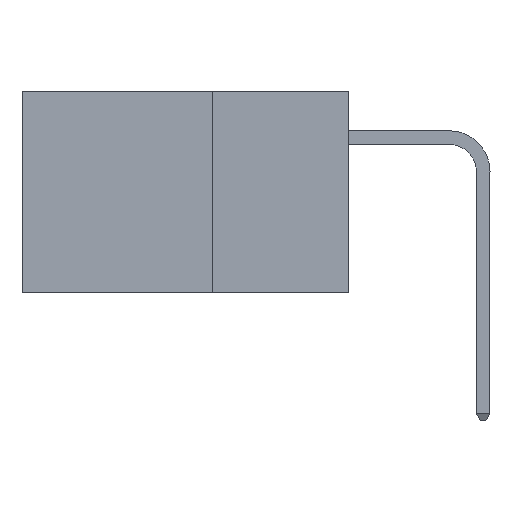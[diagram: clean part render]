
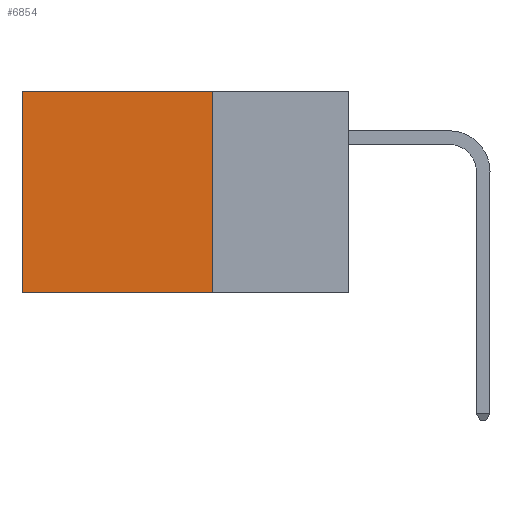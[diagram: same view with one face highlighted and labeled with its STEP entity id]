
A CAD part, left-side view. The second image highlights one B-rep face of the part: STEP entity #6854.
In plain terms, the highlighted planar face has unit normal (-1, 0, 0).
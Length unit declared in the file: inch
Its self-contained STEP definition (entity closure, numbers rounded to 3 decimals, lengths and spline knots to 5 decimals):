
#542 = FACE_OUTER_BOUND ( 'NONE', #11279, .T. ) ;
#1296 = VECTOR ( 'NONE', #21914, 39.37008 ) ;
#1816 = VECTOR ( 'NONE', #30717, 39.37008 ) ;
#2534 = VECTOR ( 'NONE', #22395, 39.37008 ) ;
#3642 = EDGE_CURVE ( 'NONE', #14192, #27919, #27334, .T. ) ;
#4705 = ORIENTED_EDGE ( 'NONE', *, *, #16904, .T. ) ;
#5171 = VERTEX_POINT ( 'NONE', #26095 ) ;
#6854 = ADVANCED_FACE ( 'NONE', ( #542 ), #18082, .F. ) ;
#7007 = VERTEX_POINT ( 'NONE', #25892 ) ;
#8223 = LINE ( 'NONE', #28835, #20538 ) ;
#8258 = DIRECTION ( 'NONE',  ( 0., 0., -1. ) ) ;
#8956 = CARTESIAN_POINT ( 'NONE',  ( 0.2875, 0.25, -0.37 ) ) ;
#11218 = CARTESIAN_POINT ( 'NONE',  ( 0.2875, 0.25, 0. ) ) ;
#11279 = EDGE_LOOP ( 'NONE', ( #28698, #12554, #26484, #4705 ) ) ;
#12554 = ORIENTED_EDGE ( 'NONE', *, *, #3642, .F. ) ;
#14192 = VERTEX_POINT ( 'NONE', #8956 ) ;
#16904 = EDGE_CURVE ( 'NONE', #5171, #7007, #26308, .T. ) ;
#17096 = CARTESIAN_POINT ( 'NONE',  ( 0.2875, 0.6, -0.37 ) ) ;
#18082 = PLANE ( 'NONE',  #29841 ) ;
#18375 = EDGE_CURVE ( 'NONE', #7007, #27919, #8223, .T. ) ;
#20520 = CARTESIAN_POINT ( 'NONE',  ( 0.2875, 0.25, 0. ) ) ;
#20538 = VECTOR ( 'NONE', #31264, 39.37008 ) ;
#21356 = LINE ( 'NONE', #27379, #2534 ) ;
#21914 = DIRECTION ( 'NONE',  ( 0., 1., 0. ) ) ;
#22395 = DIRECTION ( 'NONE',  ( 0., 0., -1. ) ) ;
#22930 = DIRECTION ( 'NONE',  ( 1., 0., 0. ) ) ;
#23438 = EDGE_CURVE ( 'NONE', #5171, #14192, #21356, .T. ) ;
#24254 = CARTESIAN_POINT ( 'NONE',  ( 0.2875, 0.25, -0.37 ) ) ;
#25892 = CARTESIAN_POINT ( 'NONE',  ( 0.2875, 0.6, 0. ) ) ;
#26095 = CARTESIAN_POINT ( 'NONE',  ( 0.2875, 0.25, 0. ) ) ;
#26308 = LINE ( 'NONE', #11218, #1816 ) ;
#26484 = ORIENTED_EDGE ( 'NONE', *, *, #23438, .F. ) ;
#27334 = LINE ( 'NONE', #24254, #1296 ) ;
#27379 = CARTESIAN_POINT ( 'NONE',  ( 0.2875, 0.25, 0. ) ) ;
#27919 = VERTEX_POINT ( 'NONE', #17096 ) ;
#28698 = ORIENTED_EDGE ( 'NONE', *, *, #18375, .T. ) ;
#28835 = CARTESIAN_POINT ( 'NONE',  ( 0.2875, 0.6, 0. ) ) ;
#29841 = AXIS2_PLACEMENT_3D ( 'NONE', #20520, #22930, #8258 ) ;
#30717 = DIRECTION ( 'NONE',  ( 0., 1., 0. ) ) ;
#31264 = DIRECTION ( 'NONE',  ( 0., 0., -1. ) ) ;
